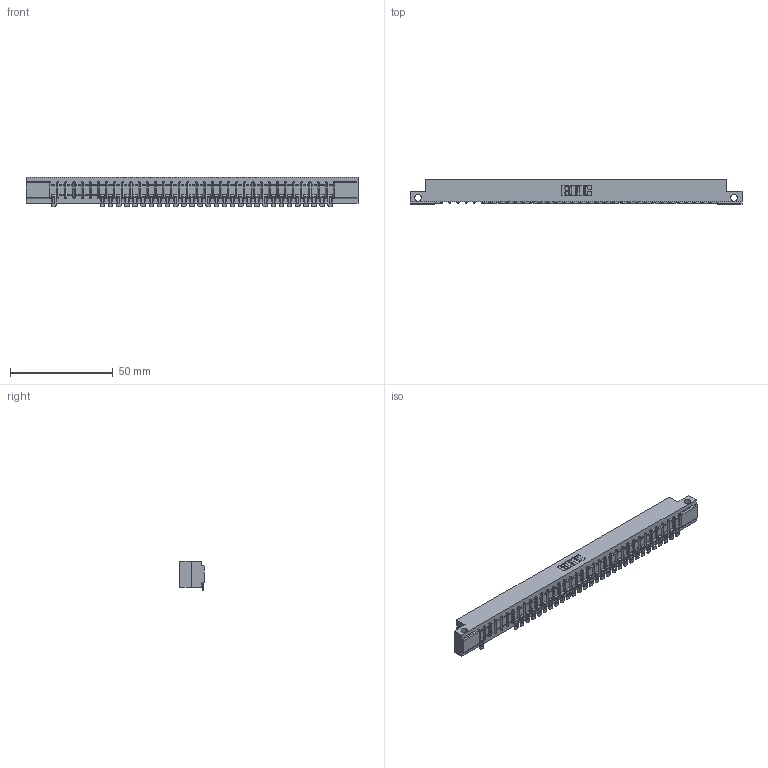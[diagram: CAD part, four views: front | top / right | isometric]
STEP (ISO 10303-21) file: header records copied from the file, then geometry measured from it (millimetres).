
FILE_DESCRIPTION (( 'STEP AP203' ), '1' );
FILE_NAME ('357-035-554-112.STEP', '2018-08-10T04:44:10', ( '' ), ( '' ), 'SwSTEP 2.0', 'SolidWorks 2016', '' );
FILE_SCHEMA (( 'CONFIG_CONTROL_DESIGN' ));
Length unit declared in the file: inch
Products named in the file (3): 307 Part_.128 Dia Side Mounting Holes; 307-290-002_554; 357-035-554-112
Assembly tree (31 placements, depth 2):
  357-035-554-112
    307 Part_.128 Dia Side Mounting Holes
    307-290-002_554  x30
Bounding box: 161.7 x 12.01 x 14.52 mm (x, y, z)
Volume: 16975.4 mm3; surface area: 20368.7 mm2
Topology: 31 solids, 31 shells, 2684 faces, 8233 edges, 5390 vertices
Faces by surface type: plane 1510, cylinder 1102, sphere 72
Entity records: 31675 total; most frequent: CARTESIAN_POINT 5365, ORIENTED_EDGE 5360, DIRECTION 5216, EDGE_CURVE 2680, LINE 2042, VECTOR 2042, VERTEX_POINT 1736, AXIS2_PLACEMENT_3D 1587
